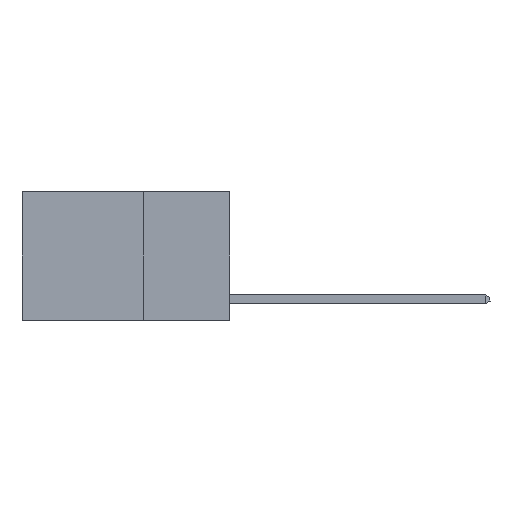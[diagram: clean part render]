
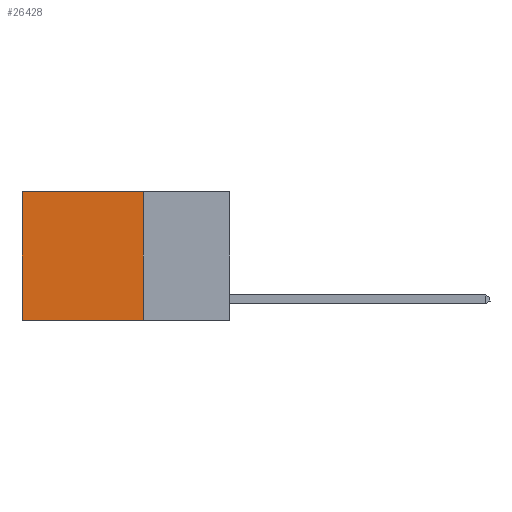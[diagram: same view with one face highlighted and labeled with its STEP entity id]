
A CAD part, left-side view. The second image highlights one B-rep face of the part: STEP entity #26428.
In plain terms, the highlighted planar face has unit normal (-1, 0, 0).
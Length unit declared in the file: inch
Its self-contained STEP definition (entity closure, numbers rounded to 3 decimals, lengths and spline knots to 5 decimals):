
#885 = LINE ( 'NONE', #19636, #6070 ) ;
#1566 = DIRECTION ( 'NONE',  ( 1., 0., 0. ) ) ;
#1666 = EDGE_CURVE ( 'NONE', #8525, #12005, #11446, .T. ) ;
#1670 = DIRECTION ( 'NONE',  ( 0., 0., -1. ) ) ;
#1955 = DIRECTION ( 'NONE',  ( 0., 1., 0. ) ) ;
#2709 = ORIENTED_EDGE ( 'NONE', *, *, #12826, .F. ) ;
#3870 = PLANE ( 'NONE',  #6337 ) ;
#5576 = VECTOR ( 'NONE', #27046, 39.37008 ) ;
#5650 = EDGE_CURVE ( 'NONE', #6132, #12005, #16803, .T. ) ;
#6070 = VECTOR ( 'NONE', #21736, 39.37008 ) ;
#6132 = VERTEX_POINT ( 'NONE', #6825 ) ;
#6337 = AXIS2_PLACEMENT_3D ( 'NONE', #14822, #1566, #1670 ) ;
#6585 = CARTESIAN_POINT ( 'NONE',  ( 0.2625, 0.6, -0.37 ) ) ;
#6825 = CARTESIAN_POINT ( 'NONE',  ( 0.2625, 0.25, -0.37 ) ) ;
#8525 = VERTEX_POINT ( 'NONE', #26536 ) ;
#8952 = LINE ( 'NONE', #25651, #25829 ) ;
#10898 = VECTOR ( 'NONE', #1955, 39.37008 ) ;
#11446 = LINE ( 'NONE', #13525, #5576 ) ;
#12005 = VERTEX_POINT ( 'NONE', #6585 ) ;
#12773 = ORIENTED_EDGE ( 'NONE', *, *, #5650, .F. ) ;
#12826 = EDGE_CURVE ( 'NONE', #13312, #6132, #885, .T. ) ;
#13092 = CARTESIAN_POINT ( 'NONE',  ( 0.2625, 0.25, -0.37 ) ) ;
#13312 = VERTEX_POINT ( 'NONE', #27476 ) ;
#13525 = CARTESIAN_POINT ( 'NONE',  ( 0.2625, 0.6, 0. ) ) ;
#13526 = ORIENTED_EDGE ( 'NONE', *, *, #28170, .T. ) ;
#14822 = CARTESIAN_POINT ( 'NONE',  ( 0.2625, 0.25, 0. ) ) ;
#15940 = EDGE_LOOP ( 'NONE', ( #19939, #12773, #2709, #13526 ) ) ;
#16803 = LINE ( 'NONE', #13092, #10898 ) ;
#19636 = CARTESIAN_POINT ( 'NONE',  ( 0.2625, 0.25, 0. ) ) ;
#19939 = ORIENTED_EDGE ( 'NONE', *, *, #1666, .T. ) ;
#21736 = DIRECTION ( 'NONE',  ( 0., 0., -1. ) ) ;
#23882 = FACE_OUTER_BOUND ( 'NONE', #15940, .T. ) ;
#25651 = CARTESIAN_POINT ( 'NONE',  ( 0.2625, 0.25, 0. ) ) ;
#25829 = VECTOR ( 'NONE', #25837, 39.37008 ) ;
#25837 = DIRECTION ( 'NONE',  ( 0., 1., 0. ) ) ;
#26428 = ADVANCED_FACE ( 'NONE', ( #23882 ), #3870, .F. ) ;
#26536 = CARTESIAN_POINT ( 'NONE',  ( 0.2625, 0.6, 0. ) ) ;
#27046 = DIRECTION ( 'NONE',  ( 0., 0., -1. ) ) ;
#27476 = CARTESIAN_POINT ( 'NONE',  ( 0.2625, 0.25, 0. ) ) ;
#28170 = EDGE_CURVE ( 'NONE', #13312, #8525, #8952, .T. ) ;
